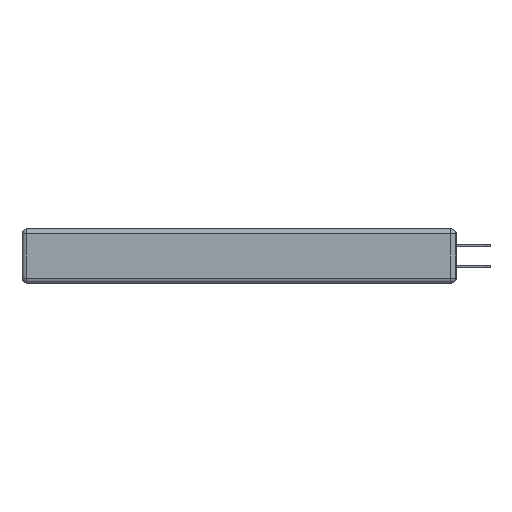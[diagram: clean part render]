
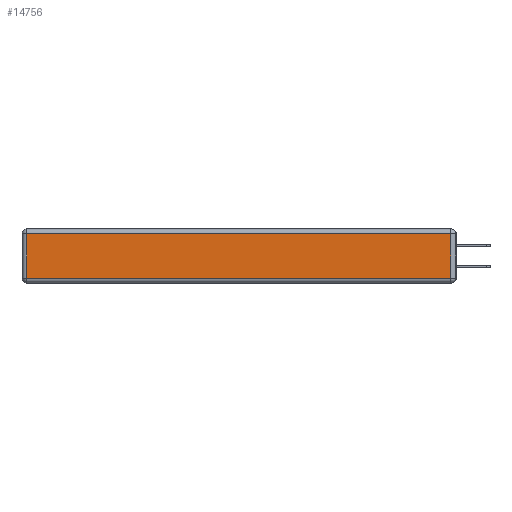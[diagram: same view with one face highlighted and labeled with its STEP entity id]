
A CAD part, left-side view. The second image highlights one B-rep face of the part: STEP entity #14756.
In plain terms, the highlighted planar face has unit normal (-1, 0, 0).
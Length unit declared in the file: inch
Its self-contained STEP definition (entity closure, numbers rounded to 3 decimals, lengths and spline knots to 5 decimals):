
#116 = EDGE_LOOP ( 'NONE', ( #858, #6849, #13338, #3116 ) ) ;
#121 = CARTESIAN_POINT ( 'NONE',  ( 0., 0.03, -0.343 ) ) ;
#858 = ORIENTED_EDGE ( 'NONE', *, *, #7041, .T. ) ;
#920 = LINE ( 'NONE', #15394, #8397 ) ;
#1453 = LINE ( 'NONE', #13012, #5001 ) ;
#2069 = LINE ( 'NONE', #10851, #5621 ) ;
#2273 = FACE_OUTER_BOUND ( 'NONE', #116, .T. ) ;
#3116 = ORIENTED_EDGE ( 'NONE', *, *, #6481, .T. ) ;
#3623 = DIRECTION ( 'NONE',  ( 0., -1., 0. ) ) ;
#4057 = DIRECTION ( 'NONE',  ( 0., 0., 1. ) ) ;
#4240 = VERTEX_POINT ( 'NONE', #13332 ) ;
#4668 = EDGE_CURVE ( 'NONE', #4240, #5658, #2069, .T. ) ;
#5001 = VECTOR ( 'NONE', #3623, 39.37008 ) ;
#5621 = VECTOR ( 'NONE', #7259, 39.37008 ) ;
#5658 = VERTEX_POINT ( 'NONE', #6412 ) ;
#5954 = VECTOR ( 'NONE', #9646, 39.37008 ) ;
#6229 = CARTESIAN_POINT ( 'NONE',  ( 0., 0.03, -0.313 ) ) ;
#6302 = DIRECTION ( 'NONE',  ( -1., 0., 0. ) ) ;
#6310 = LINE ( 'NONE', #121, #5954 ) ;
#6412 = CARTESIAN_POINT ( 'NONE',  ( 0., 2.72, -0.03 ) ) ;
#6481 = EDGE_CURVE ( 'NONE', #5658, #13322, #920, .T. ) ;
#6763 = AXIS2_PLACEMENT_3D ( 'NONE', #11037, #6302, #4057 ) ;
#6849 = ORIENTED_EDGE ( 'NONE', *, *, #10903, .T. ) ;
#7041 = EDGE_CURVE ( 'NONE', #13322, #9958, #1453, .T. ) ;
#7259 = DIRECTION ( 'NONE',  ( 0., 1., 0. ) ) ;
#8397 = VECTOR ( 'NONE', #10544, 39.37008 ) ;
#9646 = DIRECTION ( 'NONE',  ( 0., 0., 1. ) ) ;
#9958 = VERTEX_POINT ( 'NONE', #6229 ) ;
#9981 = PLANE ( 'NONE',  #6763 ) ;
#10544 = DIRECTION ( 'NONE',  ( 0., 0., -1. ) ) ;
#10851 = CARTESIAN_POINT ( 'NONE',  ( 0., 2.75, -0.03 ) ) ;
#10903 = EDGE_CURVE ( 'NONE', #9958, #4240, #6310, .T. ) ;
#11037 = CARTESIAN_POINT ( 'NONE',  ( 0., 0., -0.343 ) ) ;
#12753 = CARTESIAN_POINT ( 'NONE',  ( 0., 2.72, -0.313 ) ) ;
#13012 = CARTESIAN_POINT ( 'NONE',  ( 0., 0., -0.313 ) ) ;
#13322 = VERTEX_POINT ( 'NONE', #12753 ) ;
#13332 = CARTESIAN_POINT ( 'NONE',  ( 0., 0.03, -0.03 ) ) ;
#13338 = ORIENTED_EDGE ( 'NONE', *, *, #4668, .T. ) ;
#14756 = ADVANCED_FACE ( 'NONE', ( #2273 ), #9981, .T. ) ;
#15394 = CARTESIAN_POINT ( 'NONE',  ( 0., 2.72, -0.343 ) ) ;
